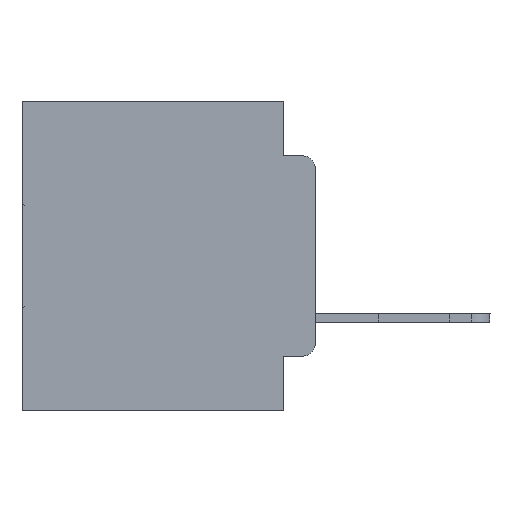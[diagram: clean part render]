
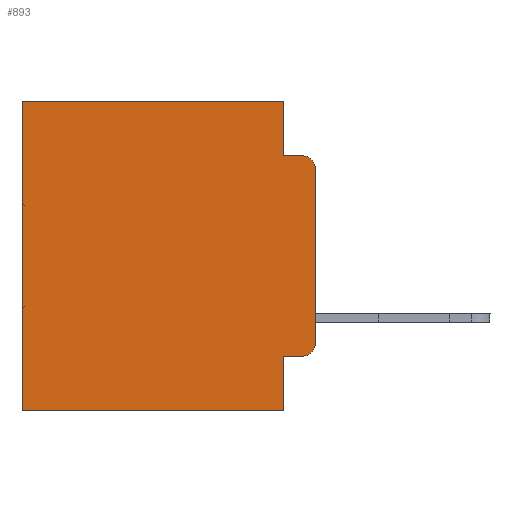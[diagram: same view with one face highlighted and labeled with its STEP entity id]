
A CAD part, left-side view. The second image highlights one B-rep face of the part: STEP entity #893.
In plain terms, the highlighted planar face has unit normal (-1, 0, 0).
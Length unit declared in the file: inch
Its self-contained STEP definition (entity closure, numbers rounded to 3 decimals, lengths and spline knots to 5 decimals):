
#18 = CARTESIAN_POINT ( 'NONE',  ( 0.298, 0.051, -0.0885 ) ) ;
#101 = EDGE_CURVE ( 'NONE', #21755, #9923, #154, .T. ) ;
#123 = CIRCLE ( 'NONE', #9205, 0.02 ) ;
#154 = LINE ( 'NONE', #29139, #15523 ) ;
#310 = EDGE_CURVE ( 'NONE', #28794, #28018, #25163, .T. ) ;
#511 = DIRECTION ( 'NONE',  ( 1., 0., 0. ) ) ;
#778 = DIRECTION ( 'NONE',  ( -1., 0., 0. ) ) ;
#893 = ADVANCED_FACE ( 'NONE', ( #24747 ), #10309, .F. ) ;
#1685 = DIRECTION ( 'NONE',  ( 0., 0., -1. ) ) ;
#1998 = VECTOR ( 'NONE', #27537, 39.37008 ) ;
#2642 = ORIENTED_EDGE ( 'NONE', *, *, #101, .T. ) ;
#3140 = DIRECTION ( 'NONE',  ( 0., 0., -1. ) ) ;
#3269 = CARTESIAN_POINT ( 'NONE',  ( 0.298, 0.051, -0.4115 ) ) ;
#3485 = EDGE_CURVE ( 'NONE', #10079, #22785, #17152, .T. ) ;
#4261 = ORIENTED_EDGE ( 'NONE', *, *, #16991, .F. ) ;
#4726 = VERTEX_POINT ( 'NONE', #13675 ) ;
#5224 = CARTESIAN_POINT ( 'NONE',  ( 0.298, 0.051, -0.5 ) ) ;
#5359 = CARTESIAN_POINT ( 'NONE',  ( 0.298, 0.051, 0. ) ) ;
#5983 = CARTESIAN_POINT ( 'NONE',  ( 0.298, 0.473, 0. ) ) ;
#6759 = LINE ( 'NONE', #23888, #16597 ) ;
#7355 = ORIENTED_EDGE ( 'NONE', *, *, #29857, .T. ) ;
#7559 = EDGE_LOOP ( 'NONE', ( #4261, #12164, #16928, #24533, #14809, #20043, #23569, #10409, #2642, #7355 ) ) ;
#7616 = CARTESIAN_POINT ( 'NONE',  ( 0.298, 0., 0. ) ) ;
#8387 = VECTOR ( 'NONE', #14441, 39.37008 ) ;
#8614 = CARTESIAN_POINT ( 'NONE',  ( 0.298, 0., 0. ) ) ;
#9205 = AXIS2_PLACEMENT_3D ( 'NONE', #9613, #18719, #13920 ) ;
#9613 = CARTESIAN_POINT ( 'NONE',  ( 0.298, 0.02, -0.3915 ) ) ;
#9724 = CARTESIAN_POINT ( 'NONE',  ( 0.298, 0.473, -0.5 ) ) ;
#9923 = VERTEX_POINT ( 'NONE', #28236 ) ;
#9975 = CARTESIAN_POINT ( 'NONE',  ( 0.298, 0.473, 0. ) ) ;
#10079 = VERTEX_POINT ( 'NONE', #18 ) ;
#10309 = PLANE ( 'NONE',  #23627 ) ;
#10409 = ORIENTED_EDGE ( 'NONE', *, *, #29949, .F. ) ;
#12164 = ORIENTED_EDGE ( 'NONE', *, *, #18461, .T. ) ;
#12307 = VECTOR ( 'NONE', #3140, 39.37008 ) ;
#13675 = CARTESIAN_POINT ( 'NONE',  ( 0.298, 0., -0.3915 ) ) ;
#13769 = LINE ( 'NONE', #25963, #18873 ) ;
#13886 = CARTESIAN_POINT ( 'NONE',  ( 0.298, 0.051, 0. ) ) ;
#13920 = DIRECTION ( 'NONE',  ( 0., 0., -1. ) ) ;
#13978 = CIRCLE ( 'NONE', #22098, 0.02 ) ;
#14441 = DIRECTION ( 'NONE',  ( 0., -1., 0. ) ) ;
#14809 = ORIENTED_EDGE ( 'NONE', *, *, #19872, .T. ) ;
#15523 = VECTOR ( 'NONE', #24550, 39.37008 ) ;
#16442 = DIRECTION ( 'NONE',  ( 0., 1., 0. ) ) ;
#16597 = VECTOR ( 'NONE', #16442, 39.37008 ) ;
#16765 = EDGE_CURVE ( 'NONE', #29627, #28018, #21810, .T. ) ;
#16928 = ORIENTED_EDGE ( 'NONE', *, *, #3485, .F. ) ;
#16991 = EDGE_CURVE ( 'NONE', #19040, #4726, #30656, .T. ) ;
#17152 = LINE ( 'NONE', #29187, #8387 ) ;
#17540 = VECTOR ( 'NONE', #1685, 39.37008 ) ;
#18461 = EDGE_CURVE ( 'NONE', #19040, #22785, #13978, .T. ) ;
#18719 = DIRECTION ( 'NONE',  ( -1., 0., 0. ) ) ;
#18855 = CARTESIAN_POINT ( 'NONE',  ( 0.298, 0.02, -0.0885 ) ) ;
#18873 = VECTOR ( 'NONE', #21085, 39.37008 ) ;
#19040 = VERTEX_POINT ( 'NONE', #19532 ) ;
#19532 = CARTESIAN_POINT ( 'NONE',  ( 0.298, 0., -0.1085 ) ) ;
#19872 = EDGE_CURVE ( 'NONE', #24563, #28794, #6759, .T. ) ;
#20043 = ORIENTED_EDGE ( 'NONE', *, *, #310, .T. ) ;
#20066 = VECTOR ( 'NONE', #31139, 39.37008 ) ;
#20157 = DIRECTION ( 'NONE',  ( 0., 0., -1. ) ) ;
#20947 = EDGE_CURVE ( 'NONE', #24563, #10079, #27069, .T. ) ;
#21085 = DIRECTION ( 'NONE',  ( 0., 0., -1. ) ) ;
#21755 = VERTEX_POINT ( 'NONE', #3269 ) ;
#21810 = LINE ( 'NONE', #29401, #20066 ) ;
#22098 = AXIS2_PLACEMENT_3D ( 'NONE', #22491, #778, #25002 ) ;
#22491 = CARTESIAN_POINT ( 'NONE',  ( 0.298, 0.02, -0.1085 ) ) ;
#22785 = VERTEX_POINT ( 'NONE', #18855 ) ;
#23569 = ORIENTED_EDGE ( 'NONE', *, *, #16765, .F. ) ;
#23627 = AXIS2_PLACEMENT_3D ( 'NONE', #7616, #511, #20157 ) ;
#23888 = CARTESIAN_POINT ( 'NONE',  ( 0.298, 0., 0. ) ) ;
#24533 = ORIENTED_EDGE ( 'NONE', *, *, #20947, .F. ) ;
#24550 = DIRECTION ( 'NONE',  ( 0., -1., 0. ) ) ;
#24563 = VERTEX_POINT ( 'NONE', #13886 ) ;
#24747 = FACE_OUTER_BOUND ( 'NONE', #7559, .T. ) ;
#25002 = DIRECTION ( 'NONE',  ( 0., 0., -1. ) ) ;
#25163 = LINE ( 'NONE', #5983, #12307 ) ;
#25963 = CARTESIAN_POINT ( 'NONE',  ( 0.298, 0.051, 0. ) ) ;
#27069 = LINE ( 'NONE', #5359, #1998 ) ;
#27537 = DIRECTION ( 'NONE',  ( 0., 0., -1. ) ) ;
#28018 = VERTEX_POINT ( 'NONE', #9724 ) ;
#28236 = CARTESIAN_POINT ( 'NONE',  ( 0.298, 0.02, -0.4115 ) ) ;
#28794 = VERTEX_POINT ( 'NONE', #9975 ) ;
#29139 = CARTESIAN_POINT ( 'NONE',  ( 0.298, 0.051, -0.4115 ) ) ;
#29187 = CARTESIAN_POINT ( 'NONE',  ( 0.298, 0.051, -0.0885 ) ) ;
#29401 = CARTESIAN_POINT ( 'NONE',  ( 0.298, 0., -0.5 ) ) ;
#29627 = VERTEX_POINT ( 'NONE', #5224 ) ;
#29857 = EDGE_CURVE ( 'NONE', #9923, #4726, #123, .T. ) ;
#29949 = EDGE_CURVE ( 'NONE', #21755, #29627, #13769, .T. ) ;
#30656 = LINE ( 'NONE', #8614, #17540 ) ;
#31139 = DIRECTION ( 'NONE',  ( 0., 1., 0. ) ) ;
